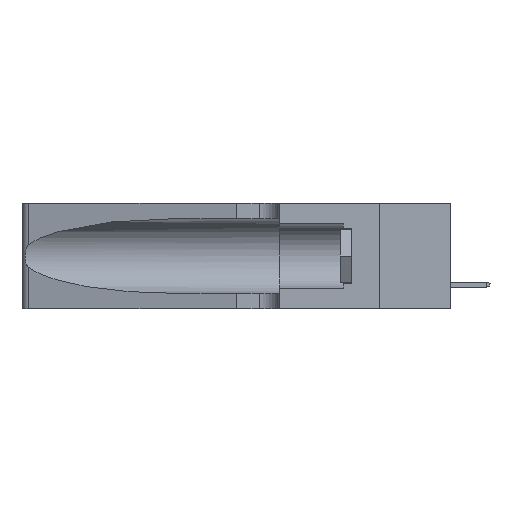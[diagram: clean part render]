
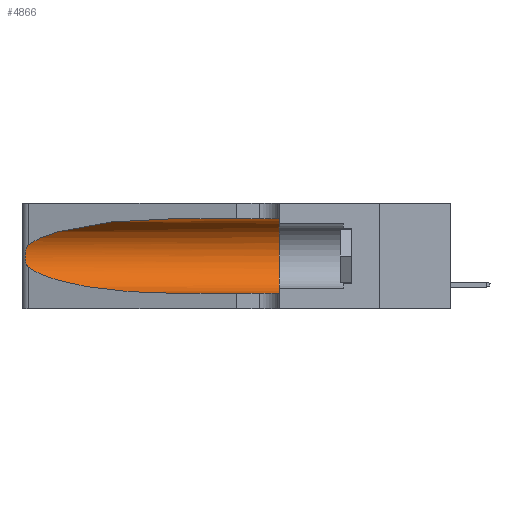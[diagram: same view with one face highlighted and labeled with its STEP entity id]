
A CAD part, left-side view. The second image highlights one B-rep face of the part: STEP entity #4866.
In plain terms, the highlighted cylindrical face has radius 3.308 mm (diameter 6.617 mm), a partial arc.
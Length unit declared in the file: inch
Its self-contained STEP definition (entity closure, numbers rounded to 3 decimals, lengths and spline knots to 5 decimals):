
#354 = CARTESIAN_POINT ( 'NONE',  ( 0.26017, 1.23833, 0.17102 ) ) ;
#488 = VECTOR ( 'NONE', #22482, 39.37008 ) ;
#897 = CARTESIAN_POINT ( 'NONE',  ( 0.25487, 1.22718, 0.14631 ) ) ;
#973 = CARTESIAN_POINT ( 'NONE',  ( 0.1305, 0.35, 0.05475 ) ) ;
#1537 =( BOUNDED_CURVE ( )  B_SPLINE_CURVE ( 3, ( #30371, #3858, #5921, #23206 ),
 .UNSPECIFIED., .F., .T. ) 
 B_SPLINE_CURVE_WITH_KNOTS ( ( 4, 4 ),
 ( 3.44316, 4.71239 ),
 .UNSPECIFIED. ) 
 CURVE ( )  GEOMETRIC_REPRESENTATION_ITEM ( )  RATIONAL_B_SPLINE_CURVE ( ( 1., 0.87, 0.87, 1. ) ) 
 REPRESENTATION_ITEM ( '' )  );
#1586 = B_SPLINE_CURVE_WITH_KNOTS ( 'NONE', 3,
 ( #17481, #26707, #17643, #29713, #15093, #27337, #22092, #12393, #354, #10018, #13652, #6217, #20968, #23342 ),
 .UNSPECIFIED., .F., .F.,
 ( 4, 2, 2, 2, 2, 2, 4 ),
 ( 0., 0.00027, 0.00053, 0.00107, 0.0016, 0.00187, 0.00214 ),
 .UNSPECIFIED. ) ;
#2562 = CIRCLE ( 'NONE', #6599, 0.13025 ) ;
#2647 = DIRECTION ( 'NONE',  ( 0., -1., 0. ) ) ;
#3303 = VERTEX_POINT ( 'NONE', #23842 ) ;
#3337 = EDGE_CURVE ( 'NONE', #21643, #3303, #13281, .T. ) ;
#3858 = CARTESIAN_POINT ( 'NONE',  ( 0.2373, 1.15595, 0.08982 ) ) ;
#4800 = CARTESIAN_POINT ( 'NONE',  ( 0.1305, 0.35, 0.185 ) ) ;
#4866 = ADVANCED_FACE ( 'NONE', ( #28526 ), #23744, .F. ) ;
#5921 = CARTESIAN_POINT ( 'NONE',  ( 0.18966, 0.96281, 0.05475 ) ) ;
#5989 = VERTEX_POINT ( 'NONE', #13170 ) ;
#6217 = CARTESIAN_POINT ( 'NONE',  ( 0.25639, 1.23186, 0.15144 ) ) ;
#6599 = AXIS2_PLACEMENT_3D ( 'NONE', #4800, #16700, #6864 ) ;
#6714 = CARTESIAN_POINT ( 'NONE',  ( 0.1305, 0.72297, 0.31525 ) ) ;
#6857 = EDGE_CURVE ( 'NONE', #31009, #5989, #1537, .T. ) ;
#6864 = DIRECTION ( 'NONE',  ( 0., 0., 1. ) ) ;
#6866 = CARTESIAN_POINT ( 'NONE',  ( 0.18966, 0.96281, 0.31525 ) ) ;
#7286 = VERTEX_POINT ( 'NONE', #973 ) ;
#7745 = LINE ( 'NONE', #29330, #488 ) ;
#8182 = ORIENTED_EDGE ( 'NONE', *, *, #27345, .T. ) ;
#8346 = EDGE_CURVE ( 'NONE', #14709, #7286, #2562, .T. ) ;
#8927 = CARTESIAN_POINT ( 'NONE',  ( 0.2373, 1.15595, 0.28018 ) ) ;
#9131 = EDGE_CURVE ( 'NONE', #21643, #14709, #7745, .T. ) ;
#9670 = VECTOR ( 'NONE', #14082, 39.37008 ) ;
#9916 = DIRECTION ( 'NONE',  ( 0., 0., -1. ) ) ;
#10018 = CARTESIAN_POINT ( 'NONE',  ( 0.25856, 1.23593, 0.16098 ) ) ;
#11534 = ORIENTED_EDGE ( 'NONE', *, *, #9131, .F. ) ;
#12274 = ORIENTED_EDGE ( 'NONE', *, *, #6857, .T. ) ;
#12393 = CARTESIAN_POINT ( 'NONE',  ( 0.26075, 1.23896, 0.178 ) ) ;
#13170 = CARTESIAN_POINT ( 'NONE',  ( 0.1305, 0.72297, 0.05475 ) ) ;
#13281 =( BOUNDED_CURVE ( )  B_SPLINE_CURVE ( 3, ( #6714, #6866, #8927, #16382 ),
 .UNSPECIFIED., .F., .F. ) 
 B_SPLINE_CURVE_WITH_KNOTS ( ( 4, 4 ),
 ( 1.5708, 2.84003 ),
 .UNSPECIFIED. ) 
 CURVE ( )  GEOMETRIC_REPRESENTATION_ITEM ( )  RATIONAL_B_SPLINE_CURVE ( ( 1., 0.87, 0.87, 1. ) ) 
 REPRESENTATION_ITEM ( '' )  );
#13652 = CARTESIAN_POINT ( 'NONE',  ( 0.25789, 1.23486, 0.15765 ) ) ;
#13925 = LINE ( 'NONE', #28235, #9670 ) ;
#14082 = DIRECTION ( 'NONE',  ( 0., -1., 0. ) ) ;
#14709 = VERTEX_POINT ( 'NONE', #26040 ) ;
#15093 = CARTESIAN_POINT ( 'NONE',  ( 0.25854, 1.2359, 0.20912 ) ) ;
#16149 = ORIENTED_EDGE ( 'NONE', *, *, #3337, .T. ) ;
#16382 = CARTESIAN_POINT ( 'NONE',  ( 0.25487, 1.22718, 0.22369 ) ) ;
#16700 = DIRECTION ( 'NONE',  ( 0., 1., 0. ) ) ;
#17432 = ORIENTED_EDGE ( 'NONE', *, *, #25519, .T. ) ;
#17481 = CARTESIAN_POINT ( 'NONE',  ( 0.25487, 1.22718, 0.22369 ) ) ;
#17643 = CARTESIAN_POINT ( 'NONE',  ( 0.25639, 1.23184, 0.21858 ) ) ;
#19459 = CARTESIAN_POINT ( 'NONE',  ( 0.1305, 1.61858, 0.185 ) ) ;
#20968 = CARTESIAN_POINT ( 'NONE',  ( 0.25555, 1.22993, 0.14849 ) ) ;
#21643 = VERTEX_POINT ( 'NONE', #24811 ) ;
#22068 = AXIS2_PLACEMENT_3D ( 'NONE', #19459, #2647, #9916 ) ;
#22092 = CARTESIAN_POINT ( 'NONE',  ( 0.26075, 1.23896, 0.19203 ) ) ;
#22259 = EDGE_LOOP ( 'NONE', ( #16149, #17432, #12274, #8182, #30041, #11534 ) ) ;
#22482 = DIRECTION ( 'NONE',  ( 0., -1., 0. ) ) ;
#23206 = CARTESIAN_POINT ( 'NONE',  ( 0.1305, 0.72297, 0.05475 ) ) ;
#23342 = CARTESIAN_POINT ( 'NONE',  ( 0.25487, 1.22718, 0.14631 ) ) ;
#23744 = CYLINDRICAL_SURFACE ( 'NONE', #22068, 0.13025 ) ;
#23842 = CARTESIAN_POINT ( 'NONE',  ( 0.25487, 1.22718, 0.22369 ) ) ;
#24811 = CARTESIAN_POINT ( 'NONE',  ( 0.1305, 0.72297, 0.31525 ) ) ;
#25519 = EDGE_CURVE ( 'NONE', #3303, #31009, #1586, .T. ) ;
#26040 = CARTESIAN_POINT ( 'NONE',  ( 0.1305, 0.35, 0.31525 ) ) ;
#26707 = CARTESIAN_POINT ( 'NONE',  ( 0.25555, 1.22994, 0.2215 ) ) ;
#27337 = CARTESIAN_POINT ( 'NONE',  ( 0.26018, 1.23835, 0.19895 ) ) ;
#27345 = EDGE_CURVE ( 'NONE', #5989, #7286, #13925, .T. ) ;
#28235 = CARTESIAN_POINT ( 'NONE',  ( 0.1305, 1.61858, 0.05475 ) ) ;
#28526 = FACE_OUTER_BOUND ( 'NONE', #22259, .T. ) ;
#29330 = CARTESIAN_POINT ( 'NONE',  ( 0.1305, 1.61858, 0.31525 ) ) ;
#29713 = CARTESIAN_POINT ( 'NONE',  ( 0.25787, 1.23484, 0.2124 ) ) ;
#30041 = ORIENTED_EDGE ( 'NONE', *, *, #8346, .F. ) ;
#30371 = CARTESIAN_POINT ( 'NONE',  ( 0.25487, 1.22718, 0.14631 ) ) ;
#31009 = VERTEX_POINT ( 'NONE', #897 ) ;
